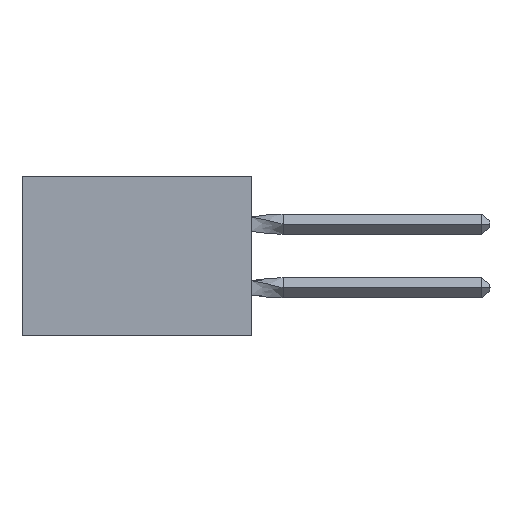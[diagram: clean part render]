
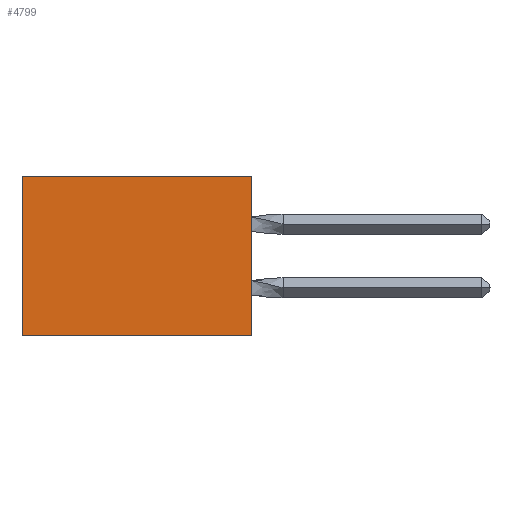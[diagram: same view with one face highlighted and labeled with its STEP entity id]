
A CAD part, left-side view. The second image highlights one B-rep face of the part: STEP entity #4799.
In plain terms, the highlighted planar face has unit normal (-1, 0, 0).
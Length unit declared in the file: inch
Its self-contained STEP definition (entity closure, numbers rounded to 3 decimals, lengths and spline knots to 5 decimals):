
#652 = EDGE_CURVE ( 'NONE', #4638, #37289, #21252, .T. ) ;
#1082 = VECTOR ( 'NONE', #45707, 39.37008 ) ;
#1133 = AXIS2_PLACEMENT_3D ( 'NONE', #37736, #12886, #19999 ) ;
#2017 = VECTOR ( 'NONE', #9914, 39.37008 ) ;
#3153 = FACE_OUTER_BOUND ( 'NONE', #25882, .T. ) ;
#3598 = VERTEX_POINT ( 'NONE', #14626 ) ;
#4206 = LINE ( 'NONE', #25429, #40869 ) ;
#4638 = VERTEX_POINT ( 'NONE', #39580 ) ;
#4799 = ADVANCED_FACE ( 'NONE', ( #3153 ), #26950, .F. ) ;
#9534 = VERTEX_POINT ( 'NONE', #16370 ) ;
#9914 = DIRECTION ( 'NONE',  ( 0., 0., -1. ) ) ;
#11630 = ORIENTED_EDGE ( 'NONE', *, *, #652, .T. ) ;
#12886 = DIRECTION ( 'NONE',  ( 1., 0., 0. ) ) ;
#13405 = EDGE_CURVE ( 'NONE', #37289, #9534, #21037, .T. ) ;
#14626 = CARTESIAN_POINT ( 'NONE',  ( 0.305, 0., -0.5 ) ) ;
#16370 = CARTESIAN_POINT ( 'NONE',  ( 0.305, 0.72, -0.5 ) ) ;
#19999 = DIRECTION ( 'NONE',  ( 0., 0., -1. ) ) ;
#20083 = EDGE_CURVE ( 'NONE', #3598, #9534, #4206, .T. ) ;
#21037 = LINE ( 'NONE', #24836, #1082 ) ;
#21072 = CARTESIAN_POINT ( 'NONE',  ( 0.305, 0., 0. ) ) ;
#21252 = LINE ( 'NONE', #21072, #41288 ) ;
#24836 = CARTESIAN_POINT ( 'NONE',  ( 0.305, 0.72, -0.5 ) ) ;
#25145 = DIRECTION ( 'NONE',  ( 0., 1., 0. ) ) ;
#25429 = CARTESIAN_POINT ( 'NONE',  ( 0.305, 0., -0.5 ) ) ;
#25882 = EDGE_LOOP ( 'NONE', ( #41913, #44775, #43293, #11630 ) ) ;
#26950 = PLANE ( 'NONE',  #1133 ) ;
#29959 = CARTESIAN_POINT ( 'NONE',  ( 0.305, 0.72, 0. ) ) ;
#30270 = LINE ( 'NONE', #44796, #2017 ) ;
#31969 = DIRECTION ( 'NONE',  ( 0., 1., 0. ) ) ;
#37289 = VERTEX_POINT ( 'NONE', #29959 ) ;
#37736 = CARTESIAN_POINT ( 'NONE',  ( 0.305, 0., -0.5 ) ) ;
#38634 = EDGE_CURVE ( 'NONE', #4638, #3598, #30270, .T. ) ;
#39580 = CARTESIAN_POINT ( 'NONE',  ( 0.305, 0., 0. ) ) ;
#40869 = VECTOR ( 'NONE', #25145, 39.37008 ) ;
#41288 = VECTOR ( 'NONE', #31969, 39.37008 ) ;
#41913 = ORIENTED_EDGE ( 'NONE', *, *, #13405, .T. ) ;
#43293 = ORIENTED_EDGE ( 'NONE', *, *, #38634, .F. ) ;
#44775 = ORIENTED_EDGE ( 'NONE', *, *, #20083, .F. ) ;
#44796 = CARTESIAN_POINT ( 'NONE',  ( 0.305, 0., -0.5 ) ) ;
#45707 = DIRECTION ( 'NONE',  ( 0., 0., -1. ) ) ;
